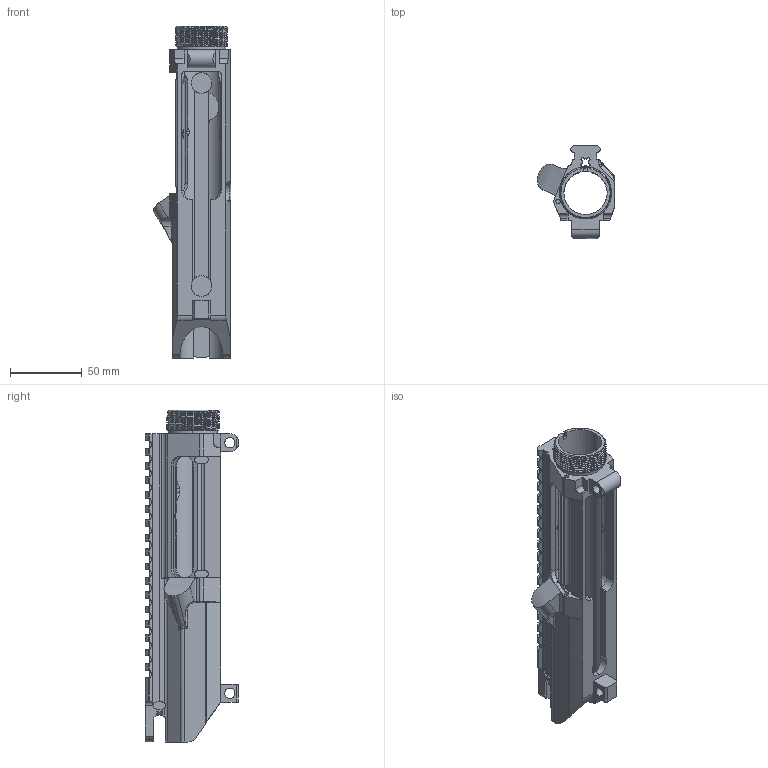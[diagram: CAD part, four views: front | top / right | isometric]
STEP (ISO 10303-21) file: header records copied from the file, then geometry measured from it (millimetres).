
FILE_DESCRIPTION (( 'STEP AP214' ), '1' );
FILE_NAME ('WX UPPER.STEP', '2016-04-23T06:01:50', ( '' ), ( '' ), 'SwSTEP 2.0', 'SolidWorks 2013', '' );
FILE_SCHEMA (( 'AUTOMOTIVE_DESIGN' ));
Length unit declared in the file: inch
Products named in the file (1): WX UPPER
Bounding box: 53.92 x 65.07 x 231.52 mm (x, y, z)
Volume: 137641.1 mm3; surface area: 66902.1 mm2
Topology: 1 solids, 1 shells, 505 faces, 1446 edges, 941 vertices
Faces by surface type: plane 285, cylinder 170, bspline 27, sphere 10, torus 9, cone 4
Entity records: 19622 total; most frequent: CARTESIAN_POINT 6798, ORIENTED_EDGE 2888, DIRECTION 2467, EDGE_CURVE 1444, VERTEX_POINT 941, LINE 923, VECTOR 923, AXIS2_PLACEMENT_3D 772
